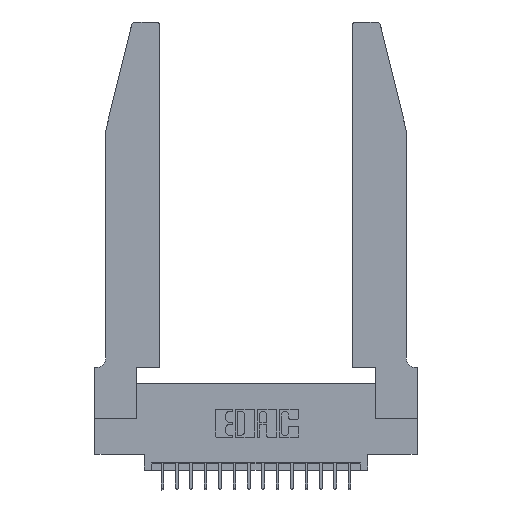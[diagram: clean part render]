
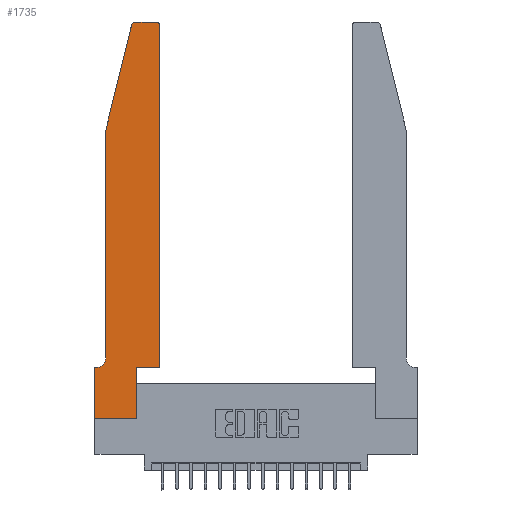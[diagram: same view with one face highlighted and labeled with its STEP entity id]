
A CAD part, top view. The second image highlights one B-rep face of the part: STEP entity #1735.
In plain terms, the highlighted planar face has unit normal (0, 0, 1).
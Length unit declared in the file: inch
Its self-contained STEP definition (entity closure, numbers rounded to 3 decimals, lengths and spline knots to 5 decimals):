
#310 = ORIENTED_EDGE ( 'NONE', *, *, #6652, .T. ) ;
#428 = DIRECTION ( 'NONE',  ( -0.239, -0.971, 0. ) ) ;
#437 = EDGE_CURVE ( 'NONE', #11739, #3612, #1712, .T. ) ;
#547 = CARTESIAN_POINT ( 'NONE',  ( 0.2865, 0., 0.37 ) ) ;
#627 = DIRECTION ( 'NONE',  ( -1., 0., 0. ) ) ;
#1096 = VECTOR ( 'NONE', #2183, 39.37008 ) ;
#1208 = AXIS2_PLACEMENT_3D ( 'NONE', #18600, #3866, #15708 ) ;
#1311 = AXIS2_PLACEMENT_3D ( 'NONE', #7324, #13392, #2429 ) ;
#1415 = DIRECTION ( 'NONE',  ( 0., 0., 1. ) ) ;
#1705 = VECTOR ( 'NONE', #2728, 39.37008 ) ;
#1712 = LINE ( 'NONE', #10794, #13617 ) ;
#1735 = ADVANCED_FACE ( 'NONE', ( #6305 ), #15455, .T. ) ;
#1896 = DIRECTION ( 'NONE',  ( 1., 0., 0. ) ) ;
#2183 = DIRECTION ( 'NONE',  ( -1., 0., 0. ) ) ;
#2244 = EDGE_CURVE ( 'NONE', #8060, #17491, #2277, .T. ) ;
#2277 = LINE ( 'NONE', #9647, #18066 ) ;
#2338 = LINE ( 'NONE', #11205, #2796 ) ;
#2429 = DIRECTION ( 'NONE',  ( 1., 0., 0. ) ) ;
#2633 = EDGE_CURVE ( 'NONE', #17491, #18696, #4429, .T. ) ;
#2728 = DIRECTION ( 'NONE',  ( 1., 0., 0. ) ) ;
#2796 = VECTOR ( 'NONE', #627, 39.37008 ) ;
#3109 = DIRECTION ( 'NONE',  ( 0., 0., 1. ) ) ;
#3144 = EDGE_CURVE ( 'NONE', #3612, #17068, #13443, .T. ) ;
#3176 = CARTESIAN_POINT ( 'NONE',  ( 0.0055, 0.35, 0.37 ) ) ;
#3382 = VERTEX_POINT ( 'NONE', #13683 ) ;
#3605 = ORIENTED_EDGE ( 'NONE', *, *, #2244, .T. ) ;
#3612 = VERTEX_POINT ( 'NONE', #8658 ) ;
#3652 = ORIENTED_EDGE ( 'NONE', *, *, #11076, .T. ) ;
#3660 = VECTOR ( 'NONE', #428, 39.37008 ) ;
#3826 = CARTESIAN_POINT ( 'NONE',  ( 0.4205, 2.75, 0.37 ) ) ;
#3866 = DIRECTION ( 'NONE',  ( 0., 0., -1. ) ) ;
#4429 = CIRCLE ( 'NONE', #1208, 0.07 ) ;
#4459 = DIRECTION ( 'NONE',  ( 1., 0., 0. ) ) ;
#4660 = EDGE_CURVE ( 'NONE', #7355, #12000, #8299, .T. ) ;
#4861 = LINE ( 'NONE', #8031, #3660 ) ;
#6233 = CIRCLE ( 'NONE', #17367, 0.03 ) ;
#6274 = ORIENTED_EDGE ( 'NONE', *, *, #437, .T. ) ;
#6305 = FACE_OUTER_BOUND ( 'NONE', #7859, .T. ) ;
#6539 = EDGE_CURVE ( 'NONE', #3382, #7355, #12763, .T. ) ;
#6652 = EDGE_CURVE ( 'NONE', #12000, #9458, #10526, .T. ) ;
#7096 = ORIENTED_EDGE ( 'NONE', *, *, #13850, .T. ) ;
#7172 = ORIENTED_EDGE ( 'NONE', *, *, #17538, .T. ) ;
#7231 = CARTESIAN_POINT ( 'NONE',  ( 0.4505, 0.35, 0.37 ) ) ;
#7280 = DIRECTION ( 'NONE',  ( 0., 1., 0. ) ) ;
#7324 = CARTESIAN_POINT ( 'NONE',  ( 0.4205, 2.72, 0.37 ) ) ;
#7334 = EDGE_CURVE ( 'NONE', #9458, #11739, #8520, .T. ) ;
#7355 = VERTEX_POINT ( 'NONE', #16389 ) ;
#7859 = EDGE_LOOP ( 'NONE', ( #7172, #3652, #14244, #3605, #11529, #7096, #16194, #14680, #310, #9935, #6274, #18281 ) ) ;
#8031 = CARTESIAN_POINT ( 'NONE',  ( 0.0755, 2., 0.37 ) ) ;
#8060 = VERTEX_POINT ( 'NONE', #19116 ) ;
#8284 = CARTESIAN_POINT ( 'NONE',  ( 0.2865, 0.35, 0.37 ) ) ;
#8299 = LINE ( 'NONE', #17364, #9292 ) ;
#8365 = EDGE_CURVE ( 'NONE', #16551, #8060, #4861, .T. ) ;
#8520 = LINE ( 'NONE', #7231, #1705 ) ;
#8658 = CARTESIAN_POINT ( 'NONE',  ( 0.4505, 2.72, 0.37 ) ) ;
#8855 = CARTESIAN_POINT ( 'NONE',  ( 0.2865, 0.35, 0.37 ) ) ;
#9013 = CARTESIAN_POINT ( 'NONE',  ( 0.284, 2.72, 0.37 ) ) ;
#9033 = VECTOR ( 'NONE', #7280, 39.37008 ) ;
#9292 = VECTOR ( 'NONE', #9679, 39.37008 ) ;
#9458 = VERTEX_POINT ( 'NONE', #8284 ) ;
#9647 = CARTESIAN_POINT ( 'NONE',  ( 0.0755, 2., 0.37 ) ) ;
#9679 = DIRECTION ( 'NONE',  ( 1., 0., 0. ) ) ;
#9935 = ORIENTED_EDGE ( 'NONE', *, *, #7334, .T. ) ;
#10526 = LINE ( 'NONE', #8855, #9033 ) ;
#10794 = CARTESIAN_POINT ( 'NONE',  ( 0.4505, 0.35, 0.37 ) ) ;
#11046 = CARTESIAN_POINT ( 'NONE',  ( 0.0755, 0.42, 0.37 ) ) ;
#11067 = CARTESIAN_POINT ( 'NONE',  ( 0., 0.35, 0.37 ) ) ;
#11076 = EDGE_CURVE ( 'NONE', #11094, #16551, #6233, .T. ) ;
#11094 = VERTEX_POINT ( 'NONE', #15788 ) ;
#11205 = CARTESIAN_POINT ( 'NONE',  ( 0.0755, 0.35, 0.37 ) ) ;
#11239 = LINE ( 'NONE', #15948, #1096 ) ;
#11529 = ORIENTED_EDGE ( 'NONE', *, *, #2633, .T. ) ;
#11739 = VERTEX_POINT ( 'NONE', #19132 ) ;
#12000 = VERTEX_POINT ( 'NONE', #547 ) ;
#12753 = DIRECTION ( 'NONE',  ( 0., -1., 0. ) ) ;
#12763 = LINE ( 'NONE', #14550, #17005 ) ;
#13392 = DIRECTION ( 'NONE',  ( 0., 0., 1. ) ) ;
#13443 = CIRCLE ( 'NONE', #1311, 0.03 ) ;
#13520 = CARTESIAN_POINT ( 'NONE',  ( 0.25487, 2.72718, 0.37 ) ) ;
#13617 = VECTOR ( 'NONE', #14291, 39.37008 ) ;
#13683 = CARTESIAN_POINT ( 'NONE',  ( 0., 0.35, 0.37 ) ) ;
#13850 = EDGE_CURVE ( 'NONE', #18696, #3382, #2338, .T. ) ;
#14244 = ORIENTED_EDGE ( 'NONE', *, *, #8365, .T. ) ;
#14291 = DIRECTION ( 'NONE',  ( 0., 1., 0. ) ) ;
#14550 = CARTESIAN_POINT ( 'NONE',  ( 0., 0., 0.37 ) ) ;
#14556 = AXIS2_PLACEMENT_3D ( 'NONE', #11067, #3109, #1896 ) ;
#14680 = ORIENTED_EDGE ( 'NONE', *, *, #4660, .T. ) ;
#15455 = PLANE ( 'NONE',  #14556 ) ;
#15708 = DIRECTION ( 'NONE',  ( -1., 0., 0. ) ) ;
#15788 = CARTESIAN_POINT ( 'NONE',  ( 0.284, 2.75, 0.37 ) ) ;
#15948 = CARTESIAN_POINT ( 'NONE',  ( 0.2605, 2.75, 0.37 ) ) ;
#16194 = ORIENTED_EDGE ( 'NONE', *, *, #6539, .T. ) ;
#16389 = CARTESIAN_POINT ( 'NONE',  ( 0., 0., 0.37 ) ) ;
#16551 = VERTEX_POINT ( 'NONE', #13520 ) ;
#17005 = VECTOR ( 'NONE', #17342, 39.37008 ) ;
#17068 = VERTEX_POINT ( 'NONE', #3826 ) ;
#17342 = DIRECTION ( 'NONE',  ( 0., -1., 0. ) ) ;
#17364 = CARTESIAN_POINT ( 'NONE',  ( 0., 0., 0.37 ) ) ;
#17367 = AXIS2_PLACEMENT_3D ( 'NONE', #9013, #1415, #4459 ) ;
#17491 = VERTEX_POINT ( 'NONE', #11046 ) ;
#17538 = EDGE_CURVE ( 'NONE', #17068, #11094, #11239, .T. ) ;
#18066 = VECTOR ( 'NONE', #12753, 39.37008 ) ;
#18281 = ORIENTED_EDGE ( 'NONE', *, *, #3144, .T. ) ;
#18600 = CARTESIAN_POINT ( 'NONE',  ( 0.0055, 0.42, 0.37 ) ) ;
#18696 = VERTEX_POINT ( 'NONE', #3176 ) ;
#19116 = CARTESIAN_POINT ( 'NONE',  ( 0.0755, 2., 0.37 ) ) ;
#19132 = CARTESIAN_POINT ( 'NONE',  ( 0.4505, 0.35, 0.37 ) ) ;
